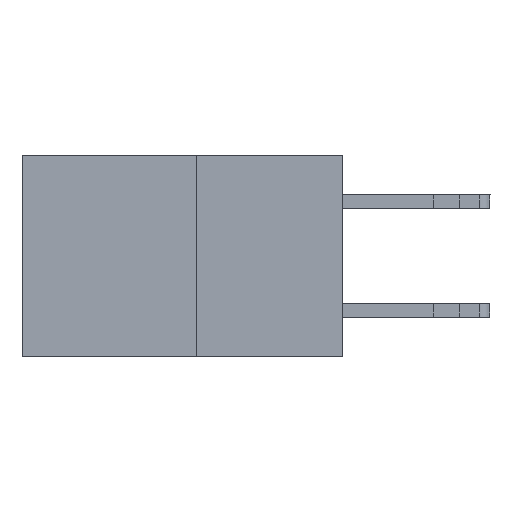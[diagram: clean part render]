
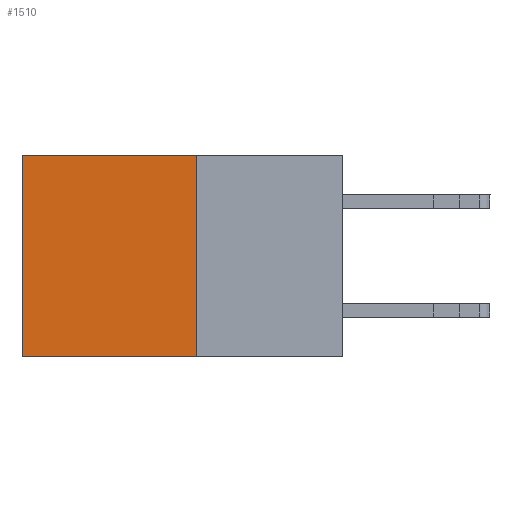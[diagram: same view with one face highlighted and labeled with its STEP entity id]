
A CAD part, left-side view. The second image highlights one B-rep face of the part: STEP entity #1510.
In plain terms, the highlighted planar face has unit normal (-1, 0, 0).
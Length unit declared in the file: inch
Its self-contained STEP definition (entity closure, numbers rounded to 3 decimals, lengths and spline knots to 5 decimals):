
#1320 = VERTEX_POINT ( 'NONE', #11717 ) ;
#1510 = ADVANCED_FACE ( 'NONE', ( #9270 ), #15738, .F. ) ;
#2270 = DIRECTION ( 'NONE',  ( 0., 1., 0. ) ) ;
#2335 = CARTESIAN_POINT ( 'NONE',  ( 0.277, 0.27, 0. ) ) ;
#3136 = EDGE_CURVE ( 'NONE', #12786, #19295, #10201, .T. ) ;
#3483 = EDGE_LOOP ( 'NONE', ( #19109, #16494, #5063, #20698 ) ) ;
#3862 = VECTOR ( 'NONE', #2270, 39.37008 ) ;
#5063 = ORIENTED_EDGE ( 'NONE', *, *, #11630, .F. ) ;
#5894 = DIRECTION ( 'NONE',  ( 0., 0., -1. ) ) ;
#6225 = CARTESIAN_POINT ( 'NONE',  ( 0.277, 0.59, 0. ) ) ;
#8340 = CARTESIAN_POINT ( 'NONE',  ( 0.277, 0.59, -0.37 ) ) ;
#8351 = EDGE_CURVE ( 'NONE', #1320, #12786, #16901, .T. ) ;
#8456 = DIRECTION ( 'NONE',  ( 0., 0., -1. ) ) ;
#9063 = CARTESIAN_POINT ( 'NONE',  ( 0.277, 0.27, -0.37 ) ) ;
#9270 = FACE_OUTER_BOUND ( 'NONE', #3483, .T. ) ;
#10201 = LINE ( 'NONE', #8340, #18297 ) ;
#10394 = LINE ( 'NONE', #15041, #18497 ) ;
#11630 = EDGE_CURVE ( 'NONE', #1320, #11712, #13640, .T. ) ;
#11712 = VERTEX_POINT ( 'NONE', #17442 ) ;
#11717 = CARTESIAN_POINT ( 'NONE',  ( 0.277, 0.27, 0. ) ) ;
#12786 = VERTEX_POINT ( 'NONE', #6225 ) ;
#13640 = LINE ( 'NONE', #9063, #17933 ) ;
#14683 = AXIS2_PLACEMENT_3D ( 'NONE', #15713, #17822, #17715 ) ;
#14787 = CARTESIAN_POINT ( 'NONE',  ( 0.277, 0.59, -0.37 ) ) ;
#15041 = CARTESIAN_POINT ( 'NONE',  ( 0.277, 0.27, -0.37 ) ) ;
#15713 = CARTESIAN_POINT ( 'NONE',  ( 0.277, 0.27, -0.37 ) ) ;
#15738 = PLANE ( 'NONE',  #14683 ) ;
#15986 = EDGE_CURVE ( 'NONE', #11712, #19295, #10394, .T. ) ;
#16494 = ORIENTED_EDGE ( 'NONE', *, *, #15986, .F. ) ;
#16680 = DIRECTION ( 'NONE',  ( 0., 1., 0. ) ) ;
#16901 = LINE ( 'NONE', #2335, #3862 ) ;
#17442 = CARTESIAN_POINT ( 'NONE',  ( 0.277, 0.27, -0.37 ) ) ;
#17715 = DIRECTION ( 'NONE',  ( 0., 0., -1. ) ) ;
#17822 = DIRECTION ( 'NONE',  ( 1., 0., 0. ) ) ;
#17933 = VECTOR ( 'NONE', #5894, 39.37008 ) ;
#18297 = VECTOR ( 'NONE', #8456, 39.37008 ) ;
#18497 = VECTOR ( 'NONE', #16680, 39.37008 ) ;
#19109 = ORIENTED_EDGE ( 'NONE', *, *, #3136, .T. ) ;
#19295 = VERTEX_POINT ( 'NONE', #14787 ) ;
#20698 = ORIENTED_EDGE ( 'NONE', *, *, #8351, .T. ) ;
